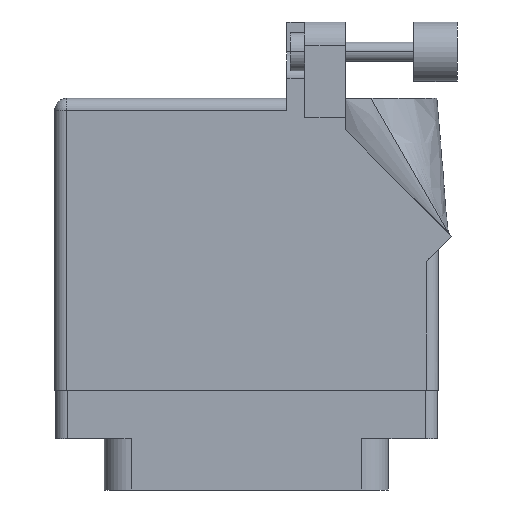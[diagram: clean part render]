
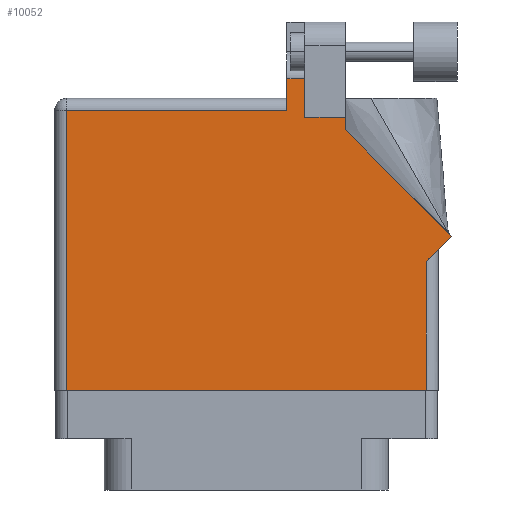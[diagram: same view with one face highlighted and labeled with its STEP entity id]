
A CAD part, front view. The second image highlights one B-rep face of the part: STEP entity #10052.
In plain terms, the highlighted face is planar.
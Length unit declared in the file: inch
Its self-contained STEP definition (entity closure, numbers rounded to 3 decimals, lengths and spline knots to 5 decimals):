
#487 = ORIENTED_EDGE ( 'NONE', *, *, #24992, .T. ) ;
#792 = CARTESIAN_POINT ( 'NONE',  ( -1.005, -0.1, 0.455 ) ) ;
#1041 = VERTEX_POINT ( 'NONE', #2191 ) ;
#1538 = DIRECTION ( 'NONE',  ( -1., 0., 0. ) ) ;
#1643 = VECTOR ( 'NONE', #17710, 39.37008 ) ;
#1685 = VECTOR ( 'NONE', #29255, 39.37008 ) ;
#1716 = ORIENTED_EDGE ( 'NONE', *, *, #28682, .T. ) ;
#2191 = CARTESIAN_POINT ( 'NONE',  ( 0.519, 1.33, 0.455 ) ) ;
#2198 = CARTESIAN_POINT ( 'NONE',  ( -0.943, -0.1, 0.455 ) ) ;
#2353 = LINE ( 'NONE', #34752, #14058 ) ;
#3010 = ORIENTED_EDGE ( 'NONE', *, *, #36383, .T. ) ;
#3130 = CARTESIAN_POINT ( 'NONE',  ( 0.943, -0.1, 0.455 ) ) ;
#4175 = CARTESIAN_POINT ( 'NONE',  ( 0.519, 1.33, 0.455 ) ) ;
#4595 = AXIS2_PLACEMENT_3D ( 'NONE', #26803, #16971, #1538 ) ;
#5278 = DIRECTION ( 'NONE',  ( -1., 0., 0. ) ) ;
#5373 = VERTEX_POINT ( 'NONE', #8399 ) ;
#6776 = LINE ( 'NONE', #25786, #9692 ) ;
#6936 = EDGE_CURVE ( 'NONE', #36494, #1041, #6776, .T. ) ;
#8399 = CARTESIAN_POINT ( 'NONE',  ( -0.943, 1.368, 0.455 ) ) ;
#8993 = VECTOR ( 'NONE', #32559, 39.37008 ) ;
#9153 = VECTOR ( 'NONE', #5278, 39.37008 ) ;
#9692 = VECTOR ( 'NONE', #35300, 39.37008 ) ;
#9821 = LINE ( 'NONE', #34203, #34733 ) ;
#10052 = ADVANCED_FACE ( 'NONE', ( #17881 ), #17258, .F. ) ;
#10172 = CARTESIAN_POINT ( 'NONE',  ( 0.519, 1.26442, 0.455 ) ) ;
#10652 = LINE ( 'NONE', #15049, #9153 ) ;
#10742 = VERTEX_POINT ( 'NONE', #14816 ) ;
#10873 = DIRECTION ( 'NONE',  ( 1., 0., 0. ) ) ;
#11147 = EDGE_CURVE ( 'NONE', #32209, #36494, #25100, .T. ) ;
#12054 = ORIENTED_EDGE ( 'NONE', *, *, #16288, .T. ) ;
#12376 = LINE ( 'NONE', #4175, #1685 ) ;
#14058 = VECTOR ( 'NONE', #32423, 39.37008 ) ;
#14080 = EDGE_CURVE ( 'NONE', #19616, #19950, #18120, .T. ) ;
#14259 = LINE ( 'NONE', #32075, #28891 ) ;
#14396 = CARTESIAN_POINT ( 'NONE',  ( -0.943, -0.1, 0.455 ) ) ;
#14675 = CARTESIAN_POINT ( 'NONE',  ( 0.306, 1.5315, 0.455 ) ) ;
#14816 = CARTESIAN_POINT ( 'NONE',  ( 0.943, 0.575, 0.455 ) ) ;
#15049 = CARTESIAN_POINT ( 'NONE',  ( 0.63677, 1.5315, 0.455 ) ) ;
#15139 = VECTOR ( 'NONE', #10873, 39.37008 ) ;
#15772 = LINE ( 'NONE', #14396, #24579 ) ;
#16288 = EDGE_CURVE ( 'NONE', #22206, #38485, #10652, .T. ) ;
#16529 = DIRECTION ( 'NONE',  ( 0., -1., 0. ) ) ;
#16971 = DIRECTION ( 'NONE',  ( 0., 0., -1. ) ) ;
#17258 = PLANE ( 'NONE',  #4595 ) ;
#17710 = DIRECTION ( 'NONE',  ( -0.707, 0.707, 0. ) ) ;
#17881 = FACE_OUTER_BOUND ( 'NONE', #18516, .T. ) ;
#18120 = LINE ( 'NONE', #792, #15139 ) ;
#18516 = EDGE_LOOP ( 'NONE', ( #28086, #12054, #1716, #487, #32049, #26791, #36784, #3010, #21928, #32659, #33781 ) ) ;
#19277 = CARTESIAN_POINT ( 'NONE',  ( 1.07571, 0.70771, 0.455 ) ) ;
#19616 = VERTEX_POINT ( 'NONE', #2198 ) ;
#19693 = DIRECTION ( 'NONE',  ( -1., 0., 0. ) ) ;
#19824 = LINE ( 'NONE', #32159, #8993 ) ;
#19950 = VERTEX_POINT ( 'NONE', #3130 ) ;
#21769 = VERTEX_POINT ( 'NONE', #21828 ) ;
#21828 = CARTESIAN_POINT ( 'NONE',  ( 0.306, 1.33, 0.455 ) ) ;
#21928 = ORIENTED_EDGE ( 'NONE', *, *, #11147, .T. ) ;
#22206 = VERTEX_POINT ( 'NONE', #14675 ) ;
#22584 = EDGE_CURVE ( 'NONE', #1041, #21769, #12376, .T. ) ;
#23042 = CARTESIAN_POINT ( 'NONE',  ( 0.212, 1.368, 0.455 ) ) ;
#23834 = CARTESIAN_POINT ( 'NONE',  ( 1.07571, 0.70771, 0.455 ) ) ;
#24579 = VECTOR ( 'NONE', #33364, 39.37008 ) ;
#24992 = EDGE_CURVE ( 'NONE', #27398, #5373, #14259, .T. ) ;
#25100 = LINE ( 'NONE', #23834, #1643 ) ;
#25405 = EDGE_CURVE ( 'NONE', #19950, #10742, #9821, .T. ) ;
#25786 = CARTESIAN_POINT ( 'NONE',  ( 0.519, 1.26442, 0.455 ) ) ;
#25844 = CARTESIAN_POINT ( 'NONE',  ( 0.212, 1.43, 0.455 ) ) ;
#26791 = ORIENTED_EDGE ( 'NONE', *, *, #14080, .T. ) ;
#26803 = CARTESIAN_POINT ( 'NONE',  ( -1.005, 1.43, 0.455 ) ) ;
#27398 = VERTEX_POINT ( 'NONE', #23042 ) ;
#28086 = ORIENTED_EDGE ( 'NONE', *, *, #36439, .T. ) ;
#28682 = EDGE_CURVE ( 'NONE', #38485, #27398, #35904, .T. ) ;
#28891 = VECTOR ( 'NONE', #19693, 39.37008 ) ;
#29255 = DIRECTION ( 'NONE',  ( -1., 0., 0. ) ) ;
#32049 = ORIENTED_EDGE ( 'NONE', *, *, #39455, .T. ) ;
#32075 = CARTESIAN_POINT ( 'NONE',  ( -1.005, 1.368, 0.455 ) ) ;
#32159 = CARTESIAN_POINT ( 'NONE',  ( 0.306, 1.33, 0.455 ) ) ;
#32209 = VERTEX_POINT ( 'NONE', #19277 ) ;
#32423 = DIRECTION ( 'NONE',  ( 0.707, 0.707, 0. ) ) ;
#32559 = DIRECTION ( 'NONE',  ( 0., 1., 0. ) ) ;
#32659 = ORIENTED_EDGE ( 'NONE', *, *, #6936, .T. ) ;
#33364 = DIRECTION ( 'NONE',  ( 0., -1., 0. ) ) ;
#33781 = ORIENTED_EDGE ( 'NONE', *, *, #22584, .T. ) ;
#34203 = CARTESIAN_POINT ( 'NONE',  ( 0.943, 0.637, 0.455 ) ) ;
#34458 = VECTOR ( 'NONE', #16529, 39.37008 ) ;
#34733 = VECTOR ( 'NONE', #37481, 39.37008 ) ;
#34752 = CARTESIAN_POINT ( 'NONE',  ( 1.005, 0.637, 0.455 ) ) ;
#35300 = DIRECTION ( 'NONE',  ( 0., 1., 0. ) ) ;
#35904 = LINE ( 'NONE', #25844, #34458 ) ;
#36383 = EDGE_CURVE ( 'NONE', #10742, #32209, #2353, .T. ) ;
#36439 = EDGE_CURVE ( 'NONE', #21769, #22206, #19824, .T. ) ;
#36494 = VERTEX_POINT ( 'NONE', #10172 ) ;
#36784 = ORIENTED_EDGE ( 'NONE', *, *, #25405, .T. ) ;
#37481 = DIRECTION ( 'NONE',  ( 0., 1., 0. ) ) ;
#38080 = CARTESIAN_POINT ( 'NONE',  ( 0.212, 1.5315, 0.455 ) ) ;
#38485 = VERTEX_POINT ( 'NONE', #38080 ) ;
#39455 = EDGE_CURVE ( 'NONE', #5373, #19616, #15772, .T. ) ;
